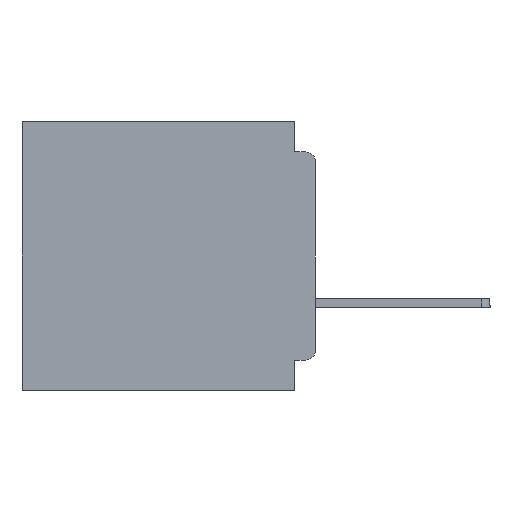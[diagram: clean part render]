
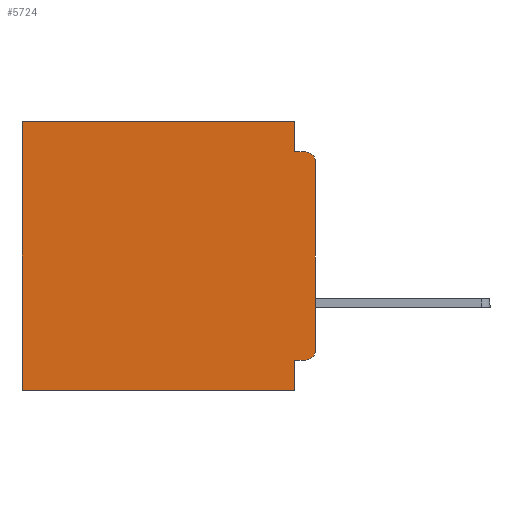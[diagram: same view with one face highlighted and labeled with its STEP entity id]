
A CAD part, left-side view. The second image highlights one B-rep face of the part: STEP entity #5724.
In plain terms, the highlighted planar face has unit normal (-1, 0, 0).
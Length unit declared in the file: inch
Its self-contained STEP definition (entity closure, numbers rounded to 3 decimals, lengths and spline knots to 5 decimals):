
#631 = VERTEX_POINT ( 'NONE', #18319 ) ;
#837 = VERTEX_POINT ( 'NONE', #53637 ) ;
#1206 = DIRECTION ( 'NONE',  ( 0., 0., -1. ) ) ;
#1691 = CARTESIAN_POINT ( 'NONE',  ( 0.3, 0.015, -0.06 ) ) ;
#2714 = DIRECTION ( 'NONE',  ( 0., 1., 0. ) ) ;
#3252 = ORIENTED_EDGE ( 'NONE', *, *, #13375, .T. ) ;
#4483 = AXIS2_PLACEMENT_3D ( 'NONE', #43139, #26387, #1206 ) ;
#5724 = ADVANCED_FACE ( 'NONE', ( #26273 ), #51513, .F. ) ;
#5856 = DIRECTION ( 'NONE',  ( 0., 0., -1. ) ) ;
#6625 = EDGE_CURVE ( 'NONE', #38731, #30165, #48412, .T. ) ;
#7802 = CARTESIAN_POINT ( 'NONE',  ( 0.3, 0., -0.4 ) ) ;
#7862 = VECTOR ( 'NONE', #24198, 39.37008 ) ;
#8023 = VECTOR ( 'NONE', #15703, 39.37008 ) ;
#8671 = CARTESIAN_POINT ( 'NONE',  ( 0.3, 0.031, -0.355 ) ) ;
#9421 = ORIENTED_EDGE ( 'NONE', *, *, #44094, .T. ) ;
#10337 = CARTESIAN_POINT ( 'NONE',  ( 0.3, 0.437, -0.4 ) ) ;
#11408 = CARTESIAN_POINT ( 'NONE',  ( 0.3, 0.031, -0.4 ) ) ;
#11921 = LINE ( 'NONE', #30932, #33047 ) ;
#12513 = LINE ( 'NONE', #34373, #33657 ) ;
#13284 = ORIENTED_EDGE ( 'NONE', *, *, #21939, .F. ) ;
#13330 = DIRECTION ( 'NONE',  ( 0., -1., 0. ) ) ;
#13375 = EDGE_CURVE ( 'NONE', #14276, #31050, #31580, .T. ) ;
#13838 = CARTESIAN_POINT ( 'NONE',  ( 0.3, 0.015, -0.34 ) ) ;
#14276 = VERTEX_POINT ( 'NONE', #33310 ) ;
#15432 = CARTESIAN_POINT ( 'NONE',  ( 0.3, 0., -0.4 ) ) ;
#15703 = DIRECTION ( 'NONE',  ( 0., 0., -1. ) ) ;
#16361 = DIRECTION ( 'NONE',  ( 0., 0., -1. ) ) ;
#17429 = ORIENTED_EDGE ( 'NONE', *, *, #6625, .T. ) ;
#18117 = DIRECTION ( 'NONE',  ( 0., 0., -1. ) ) ;
#18319 = CARTESIAN_POINT ( 'NONE',  ( 0.3, 0.015, -0.045 ) ) ;
#18588 = DIRECTION ( 'NONE',  ( 0., 1., 0. ) ) ;
#21196 = LINE ( 'NONE', #15432, #50703 ) ;
#21897 = LINE ( 'NONE', #22801, #42944 ) ;
#21939 = EDGE_CURVE ( 'NONE', #30398, #30407, #21196, .T. ) ;
#22260 = EDGE_CURVE ( 'NONE', #837, #631, #12513, .T. ) ;
#22801 = CARTESIAN_POINT ( 'NONE',  ( 0.3, 0.437, -0.4 ) ) ;
#24198 = DIRECTION ( 'NONE',  ( 0., 0., -1. ) ) ;
#25112 = ORIENTED_EDGE ( 'NONE', *, *, #49352, .F. ) ;
#25358 = CARTESIAN_POINT ( 'NONE',  ( 0.3, 0.031, 0. ) ) ;
#26084 = VECTOR ( 'NONE', #45588, 39.37008 ) ;
#26273 = FACE_OUTER_BOUND ( 'NONE', #35139, .T. ) ;
#26387 = DIRECTION ( 'NONE',  ( 1., 0., 0. ) ) ;
#27639 = LINE ( 'NONE', #7802, #48650 ) ;
#28083 = AXIS2_PLACEMENT_3D ( 'NONE', #13838, #43291, #18117 ) ;
#29985 = CARTESIAN_POINT ( 'NONE',  ( 0.3, 0.437, 0. ) ) ;
#30165 = VERTEX_POINT ( 'NONE', #29985 ) ;
#30213 = ORIENTED_EDGE ( 'NONE', *, *, #31722, .F. ) ;
#30398 = VERTEX_POINT ( 'NONE', #43872 ) ;
#30407 = VERTEX_POINT ( 'NONE', #10337 ) ;
#30932 = CARTESIAN_POINT ( 'NONE',  ( 0.3, 0., -0.355 ) ) ;
#31050 = VERTEX_POINT ( 'NONE', #36882 ) ;
#31161 = DIRECTION ( 'NONE',  ( -1., 0., 0. ) ) ;
#31580 = CIRCLE ( 'NONE', #28083, 0.015 ) ;
#31722 = EDGE_CURVE ( 'NONE', #39315, #31050, #27639, .T. ) ;
#31850 = CIRCLE ( 'NONE', #53183, 0.015 ) ;
#33047 = VECTOR ( 'NONE', #18588, 39.37008 ) ;
#33310 = CARTESIAN_POINT ( 'NONE',  ( 0.3, 0.015, -0.355 ) ) ;
#33657 = VECTOR ( 'NONE', #13330, 39.37008 ) ;
#34373 = CARTESIAN_POINT ( 'NONE',  ( 0.3, 0., -0.045 ) ) ;
#35139 = EDGE_LOOP ( 'NONE', ( #30213, #9421, #39071, #52032, #17429, #35704, #13284, #25112, #35625, #3252 ) ) ;
#35625 = ORIENTED_EDGE ( 'NONE', *, *, #41099, .F. ) ;
#35704 = ORIENTED_EDGE ( 'NONE', *, *, #40688, .T. ) ;
#36882 = CARTESIAN_POINT ( 'NONE',  ( 0.3, 0., -0.34 ) ) ;
#38731 = VERTEX_POINT ( 'NONE', #25358 ) ;
#39071 = ORIENTED_EDGE ( 'NONE', *, *, #22260, .F. ) ;
#39315 = VERTEX_POINT ( 'NONE', #51183 ) ;
#40688 = EDGE_CURVE ( 'NONE', #30165, #30407, #21897, .T. ) ;
#41099 = EDGE_CURVE ( 'NONE', #14276, #52919, #11921, .T. ) ;
#41407 = CARTESIAN_POINT ( 'NONE',  ( 0.3, 0., 0. ) ) ;
#42944 = VECTOR ( 'NONE', #47926, 39.37008 ) ;
#43139 = CARTESIAN_POINT ( 'NONE',  ( 0.3, 0., -0.4 ) ) ;
#43291 = DIRECTION ( 'NONE',  ( -1., 0., 0. ) ) ;
#43872 = CARTESIAN_POINT ( 'NONE',  ( 0.3, 0.031, -0.4 ) ) ;
#44094 = EDGE_CURVE ( 'NONE', #39315, #631, #31850, .T. ) ;
#45163 = CARTESIAN_POINT ( 'NONE',  ( 0.3, 0.031, 0. ) ) ;
#45588 = DIRECTION ( 'NONE',  ( 0., 1., 0. ) ) ;
#47926 = DIRECTION ( 'NONE',  ( 0., 0., -1. ) ) ;
#48412 = LINE ( 'NONE', #41407, #26084 ) ;
#48650 = VECTOR ( 'NONE', #16361, 39.37008 ) ;
#49352 = EDGE_CURVE ( 'NONE', #52919, #30398, #52766, .T. ) ;
#50642 = EDGE_CURVE ( 'NONE', #38731, #837, #52610, .T. ) ;
#50703 = VECTOR ( 'NONE', #2714, 39.37008 ) ;
#51183 = CARTESIAN_POINT ( 'NONE',  ( 0.3, 0., -0.06 ) ) ;
#51513 = PLANE ( 'NONE',  #4483 ) ;
#52032 = ORIENTED_EDGE ( 'NONE', *, *, #50642, .F. ) ;
#52610 = LINE ( 'NONE', #45163, #7862 ) ;
#52766 = LINE ( 'NONE', #11408, #8023 ) ;
#52919 = VERTEX_POINT ( 'NONE', #8671 ) ;
#53183 = AXIS2_PLACEMENT_3D ( 'NONE', #1691, #31161, #5856 ) ;
#53637 = CARTESIAN_POINT ( 'NONE',  ( 0.3, 0.031, -0.045 ) ) ;
